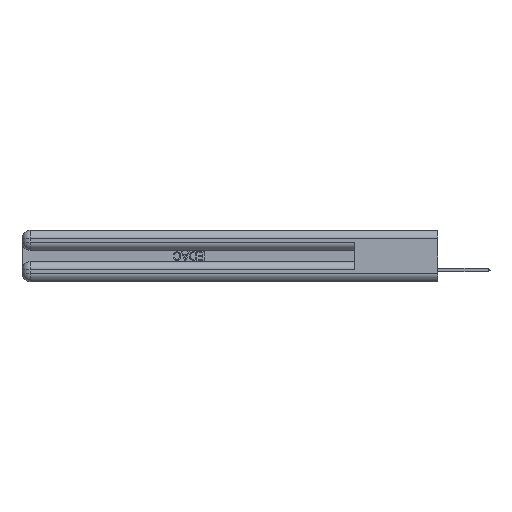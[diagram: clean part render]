
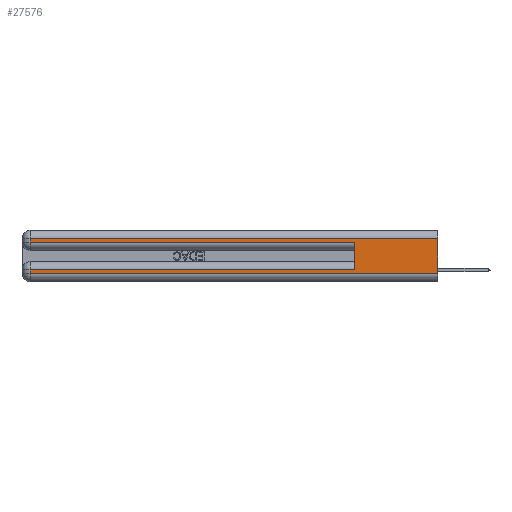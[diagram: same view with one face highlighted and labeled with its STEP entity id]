
A CAD part, left-side view. The second image highlights one B-rep face of the part: STEP entity #27576.
In plain terms, the highlighted planar face has unit normal (-1, 0, 0).
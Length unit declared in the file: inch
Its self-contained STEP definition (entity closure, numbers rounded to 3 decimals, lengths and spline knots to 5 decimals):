
#1213 = DIRECTION ( 'NONE',  ( 0., -1., 0. ) ) ;
#1914 = VECTOR ( 'NONE', #4602, 39.37008 ) ;
#2209 = EDGE_CURVE ( 'NONE', #21270, #10048, #14924, .T. ) ;
#2250 = CARTESIAN_POINT ( 'NONE',  ( 0., 2.94, 0.37 ) ) ;
#4602 = DIRECTION ( 'NONE',  ( 0., 0., -1. ) ) ;
#4889 = VERTEX_POINT ( 'NONE', #6424 ) ;
#6424 = CARTESIAN_POINT ( 'NONE',  ( 0., 0., 0.31 ) ) ;
#6603 = DIRECTION ( 'NONE',  ( 0., 0., -1. ) ) ;
#7599 = ORIENTED_EDGE ( 'NONE', *, *, #22209, .F. ) ;
#7655 = VECTOR ( 'NONE', #12927, 39.37008 ) ;
#8543 = CARTESIAN_POINT ( 'NONE',  ( 0., 0., 0.285 ) ) ;
#8570 = DIRECTION ( 'NONE',  ( 0., 1., 0. ) ) ;
#8634 = DIRECTION ( 'NONE',  ( 0., 0., -1. ) ) ;
#8870 = CARTESIAN_POINT ( 'NONE',  ( 0., 2.94, 0.285 ) ) ;
#10048 = VERTEX_POINT ( 'NONE', #8870 ) ;
#10306 = EDGE_CURVE ( 'NONE', #37277, #17795, #34003, .T. ) ;
#11636 = DIRECTION ( 'NONE',  ( 0., 0., 1. ) ) ;
#11955 = AXIS2_PLACEMENT_3D ( 'NONE', #13306, #29795, #6603 ) ;
#12745 = EDGE_LOOP ( 'NONE', ( #16400, #19921, #28435, #14033, #7599, #39167, #31202, #30040 ) ) ;
#12927 = DIRECTION ( 'NONE',  ( 0., 0., -1. ) ) ;
#13306 = CARTESIAN_POINT ( 'NONE',  ( 0., 0., 0.37 ) ) ;
#13713 = CARTESIAN_POINT ( 'NONE',  ( 0., 0.6, 0.285 ) ) ;
#14033 = ORIENTED_EDGE ( 'NONE', *, *, #27877, .T. ) ;
#14206 = CARTESIAN_POINT ( 'NONE',  ( 0., 0.6, 0.085 ) ) ;
#14924 = LINE ( 'NONE', #2250, #17584 ) ;
#16338 = CARTESIAN_POINT ( 'NONE',  ( 0., 2.94, 0.31 ) ) ;
#16400 = ORIENTED_EDGE ( 'NONE', *, *, #29422, .F. ) ;
#17277 = VECTOR ( 'NONE', #1213, 39.37008 ) ;
#17584 = VECTOR ( 'NONE', #8634, 39.37008 ) ;
#17795 = VERTEX_POINT ( 'NONE', #34410 ) ;
#18170 = VECTOR ( 'NONE', #8570, 39.37008 ) ;
#18732 = EDGE_CURVE ( 'NONE', #17795, #21045, #25431, .T. ) ;
#19921 = ORIENTED_EDGE ( 'NONE', *, *, #31564, .T. ) ;
#19991 = CARTESIAN_POINT ( 'NONE',  ( 0., 0., 0.37 ) ) ;
#20870 = CARTESIAN_POINT ( 'NONE',  ( 0., 0., 0.085 ) ) ;
#21045 = VERTEX_POINT ( 'NONE', #22326 ) ;
#21270 = VERTEX_POINT ( 'NONE', #16338 ) ;
#22209 = EDGE_CURVE ( 'NONE', #25952, #41975, #37168, .T. ) ;
#22326 = CARTESIAN_POINT ( 'NONE',  ( 0., 0., 0.06 ) ) ;
#23797 = LINE ( 'NONE', #19991, #7655 ) ;
#25111 = CARTESIAN_POINT ( 'NONE',  ( 0., 2.94, 0.37 ) ) ;
#25431 = LINE ( 'NONE', #32354, #44123 ) ;
#25812 = DIRECTION ( 'NONE',  ( 0., -1., 0. ) ) ;
#25952 = VERTEX_POINT ( 'NONE', #14206 ) ;
#26279 = LINE ( 'NONE', #30548, #34789 ) ;
#26806 = PLANE ( 'NONE',  #11955 ) ;
#26807 = LINE ( 'NONE', #20870, #18170 ) ;
#27008 = DIRECTION ( 'NONE',  ( 0., 1., 0. ) ) ;
#27576 = ADVANCED_FACE ( 'NONE', ( #30235 ), #26806, .F. ) ;
#27877 = EDGE_CURVE ( 'NONE', #10048, #41975, #29077, .T. ) ;
#28435 = ORIENTED_EDGE ( 'NONE', *, *, #2209, .T. ) ;
#29077 = LINE ( 'NONE', #8543, #17277 ) ;
#29422 = EDGE_CURVE ( 'NONE', #4889, #21045, #23797, .T. ) ;
#29795 = DIRECTION ( 'NONE',  ( 1., 0., 0. ) ) ;
#30040 = ORIENTED_EDGE ( 'NONE', *, *, #18732, .T. ) ;
#30235 = FACE_OUTER_BOUND ( 'NONE', #12745, .T. ) ;
#30548 = CARTESIAN_POINT ( 'NONE',  ( 0., 0., 0.31 ) ) ;
#31202 = ORIENTED_EDGE ( 'NONE', *, *, #10306, .T. ) ;
#31564 = EDGE_CURVE ( 'NONE', #4889, #21270, #26279, .T. ) ;
#32354 = CARTESIAN_POINT ( 'NONE',  ( 0., 0., 0.06 ) ) ;
#34003 = LINE ( 'NONE', #25111, #1914 ) ;
#34410 = CARTESIAN_POINT ( 'NONE',  ( 0., 2.94, 0.06 ) ) ;
#34778 = CARTESIAN_POINT ( 'NONE',  ( 0., 2.94, 0.085 ) ) ;
#34789 = VECTOR ( 'NONE', #27008, 39.37008 ) ;
#37128 = VECTOR ( 'NONE', #11636, 39.37008 ) ;
#37168 = LINE ( 'NONE', #38721, #37128 ) ;
#37277 = VERTEX_POINT ( 'NONE', #34778 ) ;
#38721 = CARTESIAN_POINT ( 'NONE',  ( 0., 0.6, 0.145 ) ) ;
#39167 = ORIENTED_EDGE ( 'NONE', *, *, #39436, .T. ) ;
#39436 = EDGE_CURVE ( 'NONE', #25952, #37277, #26807, .T. ) ;
#41975 = VERTEX_POINT ( 'NONE', #13713 ) ;
#44123 = VECTOR ( 'NONE', #25812, 39.37008 ) ;
